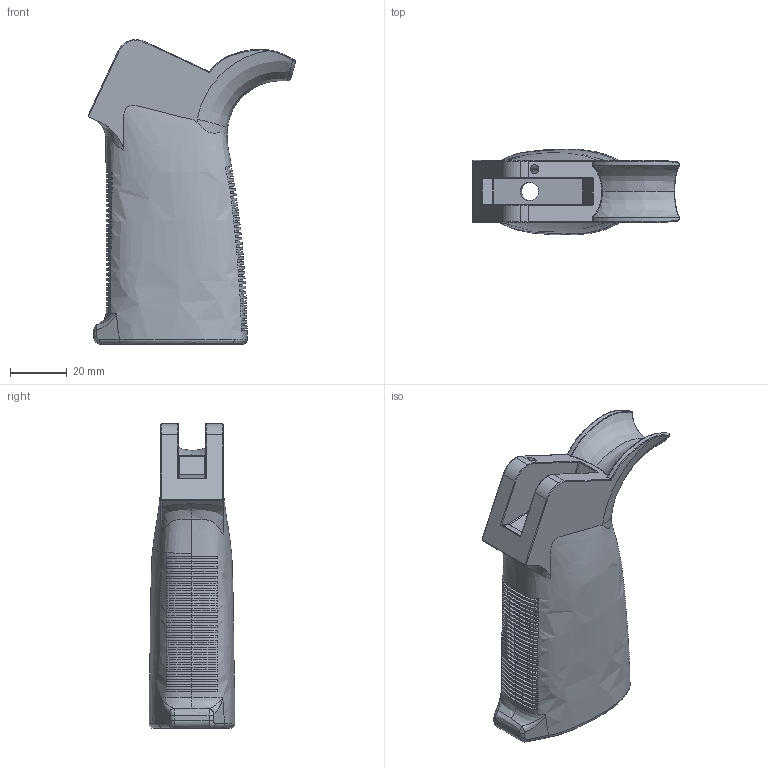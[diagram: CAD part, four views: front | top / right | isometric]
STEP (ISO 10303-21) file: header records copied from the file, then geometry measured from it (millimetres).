
FILE_DESCRIPTION (( 'STEP AP214' ), '1' );
FILE_NAME ('GRIP.STEP', '2015-09-01T23:29:54', ( '' ), ( '' ), 'SwSTEP 2.0', 'SolidWorks 2015', '' );
FILE_SCHEMA (( 'AUTOMOTIVE_DESIGN' ));
Length unit declared in the file: millimetre
Products named in the file (1): GRIP
Bounding box: 73.05 x 30.13 x 107.06 mm (x, y, z)
Volume: 80087.7 mm3; surface area: 26540.2 mm2
Topology: 1 solids, 1 shells, 529 faces, 1497 edges, 967 vertices
Faces by surface type: plane 270, bspline 205, cylinder 54
Entity records: 50208 total; most frequent: CARTESIAN_POINT 33367, ORIENTED_EDGE 2984, EDGE_CURVE 1492, DIRECTION 1251, B_SPLINE_CURVE_WITH_KNOTS 994, VERTEX_POINT 967, EDGE_LOOP 533, FACE_OUTER_BOUND 529
